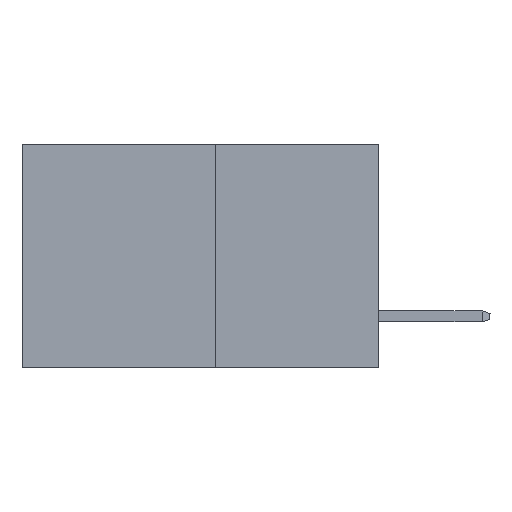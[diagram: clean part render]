
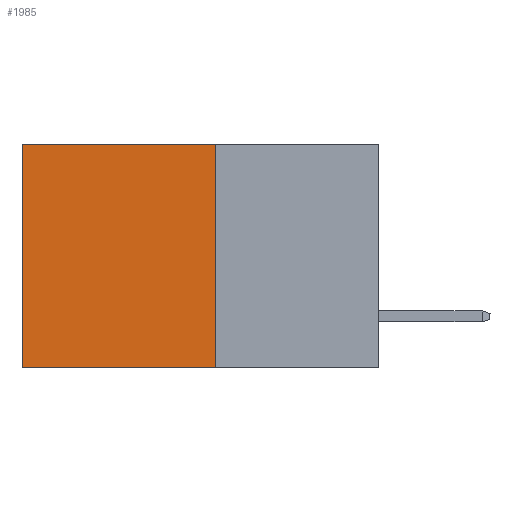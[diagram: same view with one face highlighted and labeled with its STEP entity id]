
A CAD part, left-side view. The second image highlights one B-rep face of the part: STEP entity #1985.
In plain terms, the highlighted planar face has unit normal (-1, 0, 0).
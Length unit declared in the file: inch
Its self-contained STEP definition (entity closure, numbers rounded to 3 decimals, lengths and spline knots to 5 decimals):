
#550 = CARTESIAN_POINT ( 'NONE',  ( 0.277, 0.59, -0.37 ) ) ;
#1985 = ADVANCED_FACE ( 'NONE', ( #15755 ), #17578, .F. ) ;
#2173 = VECTOR ( 'NONE', #27271, 39.37008 ) ;
#3146 = ORIENTED_EDGE ( 'NONE', *, *, #9460, .T. ) ;
#4383 = ORIENTED_EDGE ( 'NONE', *, *, #10563, .T. ) ;
#5373 = DIRECTION ( 'NONE',  ( 0., 0., -1. ) ) ;
#6342 = VECTOR ( 'NONE', #5373, 39.37008 ) ;
#6770 = VERTEX_POINT ( 'NONE', #12440 ) ;
#7043 = CARTESIAN_POINT ( 'NONE',  ( 0.277, 0.59, 0. ) ) ;
#7124 = VERTEX_POINT ( 'NONE', #7043 ) ;
#7568 = LINE ( 'NONE', #24477, #18382 ) ;
#9220 = VECTOR ( 'NONE', #20133, 39.37008 ) ;
#9460 = EDGE_CURVE ( 'NONE', #7124, #27299, #24972, .T. ) ;
#9645 = ORIENTED_EDGE ( 'NONE', *, *, #11791, .F. ) ;
#10360 = EDGE_LOOP ( 'NONE', ( #3146, #9645, #27272, #4383 ) ) ;
#10563 = EDGE_CURVE ( 'NONE', #6770, #7124, #7568, .T. ) ;
#11791 = EDGE_CURVE ( 'NONE', #25895, #27299, #21327, .T. ) ;
#12371 = CARTESIAN_POINT ( 'NONE',  ( 0.277, 0.59, -0.37 ) ) ;
#12440 = CARTESIAN_POINT ( 'NONE',  ( 0.277, 0.27, 0. ) ) ;
#15755 = FACE_OUTER_BOUND ( 'NONE', #10360, .T. ) ;
#16163 = CARTESIAN_POINT ( 'NONE',  ( 0.277, 0.27, -0.37 ) ) ;
#17578 = PLANE ( 'NONE',  #26800 ) ;
#17823 = LINE ( 'NONE', #20270, #6342 ) ;
#17859 = DIRECTION ( 'NONE',  ( 0., 0., -1. ) ) ;
#17988 = DIRECTION ( 'NONE',  ( 1., 0., 0. ) ) ;
#18382 = VECTOR ( 'NONE', #26584, 39.37008 ) ;
#20133 = DIRECTION ( 'NONE',  ( 0., 1., 0. ) ) ;
#20270 = CARTESIAN_POINT ( 'NONE',  ( 0.277, 0.27, -0.37 ) ) ;
#20881 = CARTESIAN_POINT ( 'NONE',  ( 0.277, 0.27, -0.37 ) ) ;
#21327 = LINE ( 'NONE', #22280, #9220 ) ;
#22280 = CARTESIAN_POINT ( 'NONE',  ( 0.277, 0.27, -0.37 ) ) ;
#23536 = EDGE_CURVE ( 'NONE', #6770, #25895, #17823, .T. ) ;
#24477 = CARTESIAN_POINT ( 'NONE',  ( 0.277, 0.27, 0. ) ) ;
#24972 = LINE ( 'NONE', #12371, #2173 ) ;
#25895 = VERTEX_POINT ( 'NONE', #20881 ) ;
#26584 = DIRECTION ( 'NONE',  ( 0., 1., 0. ) ) ;
#26800 = AXIS2_PLACEMENT_3D ( 'NONE', #16163, #17988, #17859 ) ;
#27271 = DIRECTION ( 'NONE',  ( 0., 0., -1. ) ) ;
#27272 = ORIENTED_EDGE ( 'NONE', *, *, #23536, .F. ) ;
#27299 = VERTEX_POINT ( 'NONE', #550 ) ;
